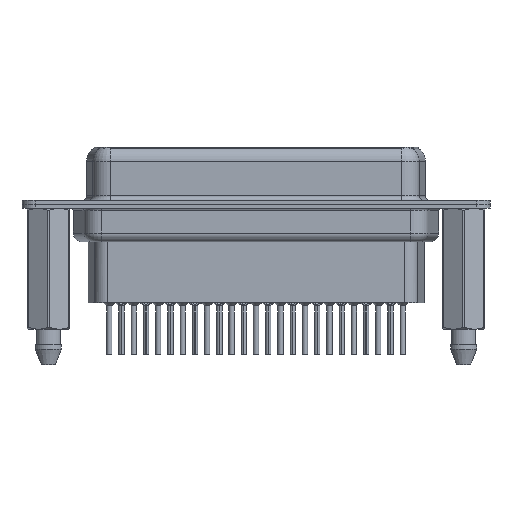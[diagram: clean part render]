
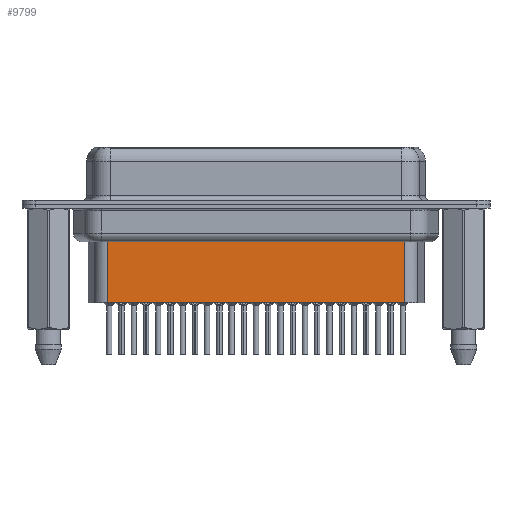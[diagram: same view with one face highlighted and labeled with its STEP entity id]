
A CAD part, front view. The second image highlights one B-rep face of the part: STEP entity #9799.
In plain terms, the highlighted planar face has unit normal (0, -1, 0).
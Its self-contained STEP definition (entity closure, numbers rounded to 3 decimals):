
#2384 = DIRECTION ( 'NONE',  ( -1., 0., 0. ) ) ;
#2474 = EDGE_LOOP ( 'NONE', ( #27237, #12647, #27691, #24141 ) ) ;
#2786 = CARTESIAN_POINT ( 'NONE',  ( 6.706, -3.5, -11.15 ) ) ;
#3520 = CARTESIAN_POINT ( 'NONE',  ( 40.344, -3.5, -11.15 ) ) ;
#4213 = VERTEX_POINT ( 'NONE', #18953 ) ;
#4454 = PLANE ( 'NONE',  #13744 ) ;
#5402 = EDGE_CURVE ( 'NONE', #4213, #17435, #26660, .T. ) ;
#5739 = CARTESIAN_POINT ( 'NONE',  ( 40.344, -3.5, -3.1 ) ) ;
#8103 = DIRECTION ( 'NONE',  ( 0., 0., -1. ) ) ;
#8636 = LINE ( 'NONE', #22171, #20451 ) ;
#9753 = VECTOR ( 'NONE', #8103, 1000. ) ;
#9799 = ADVANCED_FACE ( 'NONE', ( #15477 ), #4454, .T. ) ;
#10395 = VECTOR ( 'NONE', #2384, 1000. ) ;
#11519 = DIRECTION ( 'NONE',  ( 0., -1., 0. ) ) ;
#11539 = VERTEX_POINT ( 'NONE', #3520 ) ;
#12647 = ORIENTED_EDGE ( 'NONE', *, *, #13782, .T. ) ;
#13039 = DIRECTION ( 'NONE',  ( -1., 0., 0. ) ) ;
#13576 = DIRECTION ( 'NONE',  ( 1., 0., 0. ) ) ;
#13744 = AXIS2_PLACEMENT_3D ( 'NONE', #22714, #11519, #13576 ) ;
#13782 = EDGE_CURVE ( 'NONE', #19905, #4213, #8636, .T. ) ;
#15453 = CARTESIAN_POINT ( 'NONE',  ( 6.706, -3.5, -3.1 ) ) ;
#15477 = FACE_OUTER_BOUND ( 'NONE', #2474, .T. ) ;
#17435 = VERTEX_POINT ( 'NONE', #2786 ) ;
#18007 = LINE ( 'NONE', #26820, #10395 ) ;
#18953 = CARTESIAN_POINT ( 'NONE',  ( 6.706, -3.5, -4.097 ) ) ;
#19798 = VECTOR ( 'NONE', #24467, 1000. ) ;
#19905 = VERTEX_POINT ( 'NONE', #27268 ) ;
#20451 = VECTOR ( 'NONE', #13039, 1000. ) ;
#20473 = EDGE_CURVE ( 'NONE', #19905, #11539, #21943, .T. ) ;
#21943 = LINE ( 'NONE', #5739, #9753 ) ;
#22171 = CARTESIAN_POINT ( 'NONE',  ( 6.459, -3.5, -4.097 ) ) ;
#22714 = CARTESIAN_POINT ( 'NONE',  ( 6.706, -3.5, -3.1 ) ) ;
#24141 = ORIENTED_EDGE ( 'NONE', *, *, #27549, .F. ) ;
#24467 = DIRECTION ( 'NONE',  ( 0., 0., -1. ) ) ;
#26660 = LINE ( 'NONE', #15453, #19798 ) ;
#26820 = CARTESIAN_POINT ( 'NONE',  ( 6.706, -3.5, -11.15 ) ) ;
#27237 = ORIENTED_EDGE ( 'NONE', *, *, #20473, .F. ) ;
#27268 = CARTESIAN_POINT ( 'NONE',  ( 40.344, -3.5, -4.097 ) ) ;
#27549 = EDGE_CURVE ( 'NONE', #11539, #17435, #18007, .T. ) ;
#27691 = ORIENTED_EDGE ( 'NONE', *, *, #5402, .T. ) ;
